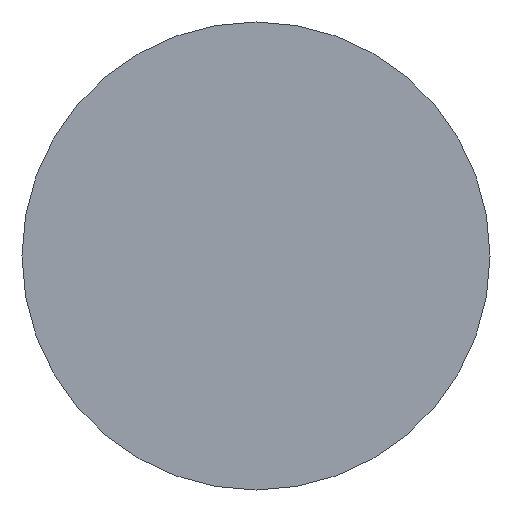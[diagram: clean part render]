
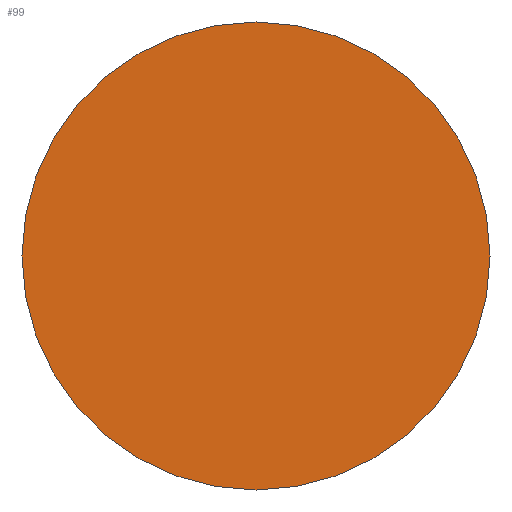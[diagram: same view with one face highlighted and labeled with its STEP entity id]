
A CAD part, front view. The second image highlights one B-rep face of the part: STEP entity #99.
In plain terms, the highlighted planar face has unit normal (0, -1, 0).
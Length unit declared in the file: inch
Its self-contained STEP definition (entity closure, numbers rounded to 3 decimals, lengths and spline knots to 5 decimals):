
#2 = DIRECTION ( 'NONE',  ( 0., -1., 0. ) ) ;
#3 = CARTESIAN_POINT ( 'NONE',  ( 0., 0., 0.15 ) ) ;
#21 = EDGE_CURVE ( 'NONE', #63, #109, #44, .T. ) ;
#24 = DIRECTION ( 'NONE',  ( 0., 0., -1. ) ) ;
#30 = EDGE_LOOP ( 'NONE', ( #120, #134 ) ) ;
#39 = DIRECTION ( 'NONE',  ( 0., -1., 0. ) ) ;
#44 = CIRCLE ( 'NONE', #59, 0.15 ) ;
#59 = AXIS2_PLACEMENT_3D ( 'NONE', #95, #103, #24 ) ;
#62 = AXIS2_PLACEMENT_3D ( 'NONE', #119, #2, #107 ) ;
#63 = VERTEX_POINT ( 'NONE', #105 ) ;
#81 = CIRCLE ( 'NONE', #62, 0.15 ) ;
#95 = CARTESIAN_POINT ( 'NONE',  ( 0., 0., 0. ) ) ;
#99 = ADVANCED_FACE ( 'NONE', ( #108 ), #131, .T. ) ;
#101 = EDGE_CURVE ( 'NONE', #109, #63, #81, .T. ) ;
#103 = DIRECTION ( 'NONE',  ( 0., -1., 0. ) ) ;
#105 = CARTESIAN_POINT ( 'NONE',  ( 0., 0., -0.15 ) ) ;
#107 = DIRECTION ( 'NONE',  ( 0., 0., -1. ) ) ;
#108 = FACE_OUTER_BOUND ( 'NONE', #30, .T. ) ;
#109 = VERTEX_POINT ( 'NONE', #3 ) ;
#110 = DIRECTION ( 'NONE',  ( 0., 0., -1. ) ) ;
#119 = CARTESIAN_POINT ( 'NONE',  ( 0., 0., 0. ) ) ;
#120 = ORIENTED_EDGE ( 'NONE', *, *, #21, .T. ) ;
#125 = AXIS2_PLACEMENT_3D ( 'NONE', #130, #39, #110 ) ;
#130 = CARTESIAN_POINT ( 'NONE',  ( 0., 0., 0. ) ) ;
#131 = PLANE ( 'NONE',  #125 ) ;
#134 = ORIENTED_EDGE ( 'NONE', *, *, #101, .T. ) ;
